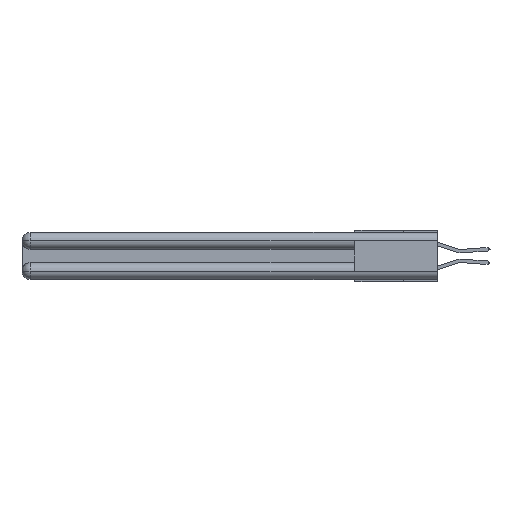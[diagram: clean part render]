
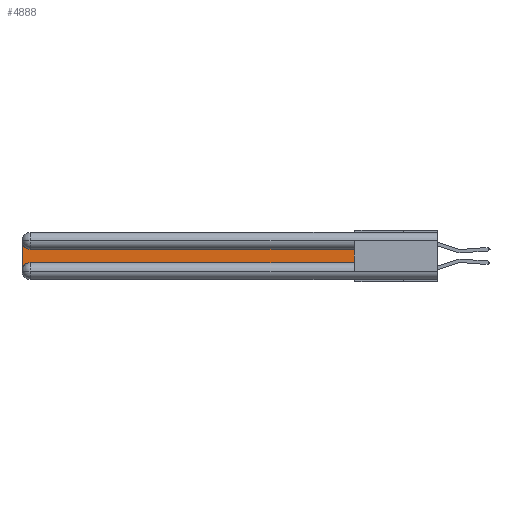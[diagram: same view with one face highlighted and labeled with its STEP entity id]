
A CAD part, left-side view. The second image highlights one B-rep face of the part: STEP entity #4888.
In plain terms, the highlighted planar face has unit normal (-1, 0, 0).
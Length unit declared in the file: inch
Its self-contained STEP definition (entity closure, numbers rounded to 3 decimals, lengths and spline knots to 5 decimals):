
#150 = ORIENTED_EDGE ( 'NONE', *, *, #31061, .T. ) ;
#598 = DIRECTION ( 'NONE',  ( 1., 0., 0. ) ) ;
#1123 = CARTESIAN_POINT ( 'NONE',  ( 0.075, 2.94, -0.1225 ) ) ;
#2183 = DIRECTION ( 'NONE',  ( 0., 1., 0. ) ) ;
#2267 = AXIS2_PLACEMENT_3D ( 'NONE', #8900, #598, #9017 ) ;
#2430 = EDGE_LOOP ( 'NONE', ( #15295, #10272, #3986, #150, #30522, #16108 ) ) ;
#3986 = ORIENTED_EDGE ( 'NONE', *, *, #18600, .T. ) ;
#4888 = ADVANCED_FACE ( 'NONE', ( #7246 ), #7962, .F. ) ;
#4958 = DIRECTION ( 'NONE',  ( 0., 0., -1. ) ) ;
#5047 = DIRECTION ( 'NONE',  ( 1., 0., 0. ) ) ;
#5105 = VERTEX_POINT ( 'NONE', #11110 ) ;
#5686 = CARTESIAN_POINT ( 'NONE',  ( 0.075, 0.6, -0.2175 ) ) ;
#5980 = VERTEX_POINT ( 'NONE', #17259 ) ;
#6196 = CARTESIAN_POINT ( 'NONE',  ( 0.075, 0.6, -0.2175 ) ) ;
#6354 = AXIS2_PLACEMENT_3D ( 'NONE', #20682, #18096, #29414 ) ;
#7246 = FACE_OUTER_BOUND ( 'NONE', #2430, .T. ) ;
#7397 = VERTEX_POINT ( 'NONE', #6196 ) ;
#7451 = VECTOR ( 'NONE', #24404, 39.37008 ) ;
#7962 = PLANE ( 'NONE',  #28645 ) ;
#8220 = CIRCLE ( 'NONE', #2267, 0.06 ) ;
#8651 = EDGE_CURVE ( 'NONE', #27166, #10870, #33379, .T. ) ;
#8900 = CARTESIAN_POINT ( 'NONE',  ( 0.075, 2.94, -0.0625 ) ) ;
#9017 = DIRECTION ( 'NONE',  ( 0., 0., -1. ) ) ;
#10272 = ORIENTED_EDGE ( 'NONE', *, *, #29449, .T. ) ;
#10870 = VERTEX_POINT ( 'NONE', #1123 ) ;
#11110 = CARTESIAN_POINT ( 'NONE',  ( 0.075, 3., -0.0625 ) ) ;
#11274 = CARTESIAN_POINT ( 'NONE',  ( 0.075, 0.6, -0.1225 ) ) ;
#14044 = EDGE_CURVE ( 'NONE', #5980, #7397, #32506, .T. ) ;
#14977 = CIRCLE ( 'NONE', #6354, 0.06 ) ;
#15295 = ORIENTED_EDGE ( 'NONE', *, *, #8651, .T. ) ;
#16108 = ORIENTED_EDGE ( 'NONE', *, *, #26073, .T. ) ;
#17259 = CARTESIAN_POINT ( 'NONE',  ( 0.075, 2.94, -0.2175 ) ) ;
#18096 = DIRECTION ( 'NONE',  ( 1., 0., 0. ) ) ;
#18333 = CARTESIAN_POINT ( 'NONE',  ( 0.075, 3., -0.1225 ) ) ;
#18600 = EDGE_CURVE ( 'NONE', #5105, #29229, #28724, .T. ) ;
#18933 = CARTESIAN_POINT ( 'NONE',  ( 0.075, 3., -0.2775 ) ) ;
#19071 = VECTOR ( 'NONE', #26566, 39.37008 ) ;
#20682 = CARTESIAN_POINT ( 'NONE',  ( 0.075, 2.94, -0.2775 ) ) ;
#21642 = VECTOR ( 'NONE', #2183, 39.37008 ) ;
#23760 = DIRECTION ( 'NONE',  ( 0., 0., -1. ) ) ;
#24404 = DIRECTION ( 'NONE',  ( 0., 0., 1. ) ) ;
#26073 = EDGE_CURVE ( 'NONE', #7397, #27166, #29709, .T. ) ;
#26566 = DIRECTION ( 'NONE',  ( 0., -1., 0. ) ) ;
#27166 = VERTEX_POINT ( 'NONE', #11274 ) ;
#28645 = AXIS2_PLACEMENT_3D ( 'NONE', #18333, #5047, #23760 ) ;
#28668 = CARTESIAN_POINT ( 'NONE',  ( 0.075, 0.6, -0.1225 ) ) ;
#28724 = LINE ( 'NONE', #31746, #32480 ) ;
#29229 = VERTEX_POINT ( 'NONE', #18933 ) ;
#29414 = DIRECTION ( 'NONE',  ( 0., 0., -1. ) ) ;
#29449 = EDGE_CURVE ( 'NONE', #10870, #5105, #8220, .T. ) ;
#29709 = LINE ( 'NONE', #5686, #7451 ) ;
#30522 = ORIENTED_EDGE ( 'NONE', *, *, #14044, .T. ) ;
#31061 = EDGE_CURVE ( 'NONE', #29229, #5980, #14977, .T. ) ;
#31746 = CARTESIAN_POINT ( 'NONE',  ( 0.075, 3., -0.2175 ) ) ;
#32480 = VECTOR ( 'NONE', #4958, 39.37008 ) ;
#32506 = LINE ( 'NONE', #33832, #19071 ) ;
#33379 = LINE ( 'NONE', #28668, #21642 ) ;
#33832 = CARTESIAN_POINT ( 'NONE',  ( 0.075, 0.6, -0.2175 ) ) ;
